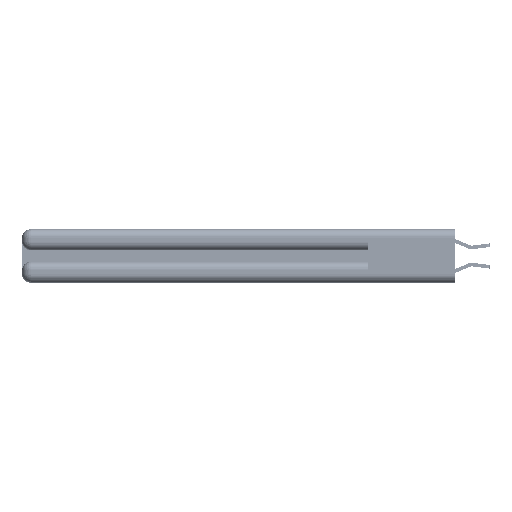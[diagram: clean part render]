
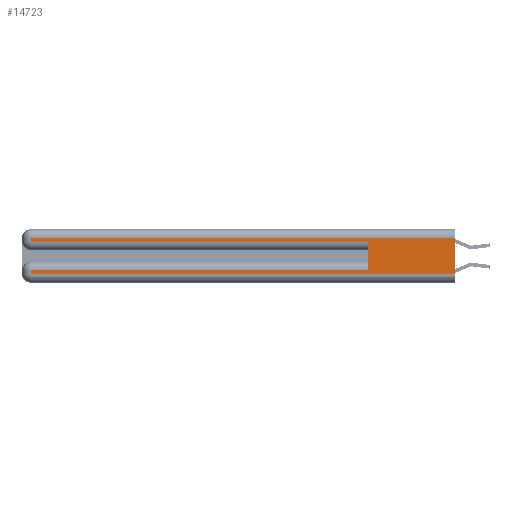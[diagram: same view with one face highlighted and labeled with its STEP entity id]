
A CAD part, left-side view. The second image highlights one B-rep face of the part: STEP entity #14723.
In plain terms, the highlighted planar face has unit normal (-1, 0, 0).
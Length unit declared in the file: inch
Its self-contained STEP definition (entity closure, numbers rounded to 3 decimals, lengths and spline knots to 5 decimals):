
#235 = LINE ( 'NONE', #29263, #10208 ) ;
#687 = ORIENTED_EDGE ( 'NONE', *, *, #10361, .T. ) ;
#1610 = CARTESIAN_POINT ( 'NONE',  ( 0., 2.94, 0.06 ) ) ;
#1762 = AXIS2_PLACEMENT_3D ( 'NONE', #10411, #19256, #21673 ) ;
#3569 = DIRECTION ( 'NONE',  ( 0., 0., 1. ) ) ;
#3870 = CARTESIAN_POINT ( 'NONE',  ( 0., 0., 0.06 ) ) ;
#4331 = CARTESIAN_POINT ( 'NONE',  ( 0., 0., 0.31 ) ) ;
#4814 = LINE ( 'NONE', #35301, #12497 ) ;
#5227 = PLANE ( 'NONE',  #1762 ) ;
#6048 = VERTEX_POINT ( 'NONE', #3870 ) ;
#6277 = VECTOR ( 'NONE', #28723, 39.37008 ) ;
#6961 = VECTOR ( 'NONE', #18670, 39.37008 ) ;
#7392 = CARTESIAN_POINT ( 'NONE',  ( 0., 0., 0.31 ) ) ;
#7670 = VERTEX_POINT ( 'NONE', #22877 ) ;
#8727 = EDGE_CURVE ( 'NONE', #21401, #6048, #20757, .T. ) ;
#8769 = VERTEX_POINT ( 'NONE', #32936 ) ;
#10208 = VECTOR ( 'NONE', #3569, 39.37008 ) ;
#10361 = EDGE_CURVE ( 'NONE', #26329, #7670, #27197, .T. ) ;
#10411 = CARTESIAN_POINT ( 'NONE',  ( 0., 0., 0.37 ) ) ;
#10543 = DIRECTION ( 'NONE',  ( 0., 1., 0. ) ) ;
#12447 = VECTOR ( 'NONE', #14994, 39.37008 ) ;
#12497 = VECTOR ( 'NONE', #15534, 39.37008 ) ;
#13702 = EDGE_CURVE ( 'NONE', #7670, #25701, #16628, .T. ) ;
#14043 = VERTEX_POINT ( 'NONE', #28996 ) ;
#14153 = ORIENTED_EDGE ( 'NONE', *, *, #13702, .T. ) ;
#14239 = LINE ( 'NONE', #19964, #19145 ) ;
#14723 = ADVANCED_FACE ( 'NONE', ( #33128 ), #5227, .F. ) ;
#14969 = EDGE_CURVE ( 'NONE', #8769, #21401, #18131, .T. ) ;
#14994 = DIRECTION ( 'NONE',  ( 0., 0., -1. ) ) ;
#15534 = DIRECTION ( 'NONE',  ( 0., 0., -1. ) ) ;
#15717 = CARTESIAN_POINT ( 'NONE',  ( 0., 2.94, 0.37 ) ) ;
#16628 = LINE ( 'NONE', #24954, #35956 ) ;
#17570 = EDGE_CURVE ( 'NONE', #14043, #35380, #235, .T. ) ;
#18131 = LINE ( 'NONE', #15717, #12447 ) ;
#18670 = DIRECTION ( 'NONE',  ( 0., 1., 0. ) ) ;
#19145 = VECTOR ( 'NONE', #31232, 39.37008 ) ;
#19256 = DIRECTION ( 'NONE',  ( 1., 0., 0. ) ) ;
#19964 = CARTESIAN_POINT ( 'NONE',  ( 0., 0., 0.285 ) ) ;
#20757 = LINE ( 'NONE', #32028, #6277 ) ;
#20929 = EDGE_CURVE ( 'NONE', #14043, #8769, #27363, .T. ) ;
#21401 = VERTEX_POINT ( 'NONE', #1610 ) ;
#21673 = DIRECTION ( 'NONE',  ( 0., 0., -1. ) ) ;
#21887 = ORIENTED_EDGE ( 'NONE', *, *, #35513, .T. ) ;
#22173 = DIRECTION ( 'NONE',  ( 0., 0., -1. ) ) ;
#22877 = CARTESIAN_POINT ( 'NONE',  ( 0., 2.94, 0.31 ) ) ;
#23595 = ORIENTED_EDGE ( 'NONE', *, *, #8727, .T. ) ;
#24398 = CARTESIAN_POINT ( 'NONE',  ( 0., 0., 0.085 ) ) ;
#24954 = CARTESIAN_POINT ( 'NONE',  ( 0., 2.94, 0.37 ) ) ;
#25662 = ORIENTED_EDGE ( 'NONE', *, *, #30347, .F. ) ;
#25701 = VERTEX_POINT ( 'NONE', #27200 ) ;
#26329 = VERTEX_POINT ( 'NONE', #4331 ) ;
#27197 = LINE ( 'NONE', #7392, #6961 ) ;
#27200 = CARTESIAN_POINT ( 'NONE',  ( 0., 2.94, 0.285 ) ) ;
#27363 = LINE ( 'NONE', #24398, #29256 ) ;
#27866 = ORIENTED_EDGE ( 'NONE', *, *, #20929, .T. ) ;
#28723 = DIRECTION ( 'NONE',  ( 0., -1., 0. ) ) ;
#28996 = CARTESIAN_POINT ( 'NONE',  ( 0., 0.6, 0.085 ) ) ;
#29256 = VECTOR ( 'NONE', #10543, 39.37008 ) ;
#29263 = CARTESIAN_POINT ( 'NONE',  ( 0., 0.6, 0.145 ) ) ;
#30347 = EDGE_CURVE ( 'NONE', #26329, #6048, #4814, .T. ) ;
#31232 = DIRECTION ( 'NONE',  ( 0., -1., 0. ) ) ;
#32028 = CARTESIAN_POINT ( 'NONE',  ( 0., 0., 0.06 ) ) ;
#32381 = EDGE_LOOP ( 'NONE', ( #25662, #687, #14153, #21887, #35373, #27866, #33283, #23595 ) ) ;
#32550 = CARTESIAN_POINT ( 'NONE',  ( 0., 0.6, 0.285 ) ) ;
#32936 = CARTESIAN_POINT ( 'NONE',  ( 0., 2.94, 0.085 ) ) ;
#33128 = FACE_OUTER_BOUND ( 'NONE', #32381, .T. ) ;
#33283 = ORIENTED_EDGE ( 'NONE', *, *, #14969, .T. ) ;
#35301 = CARTESIAN_POINT ( 'NONE',  ( 0., 0., 0.37 ) ) ;
#35373 = ORIENTED_EDGE ( 'NONE', *, *, #17570, .F. ) ;
#35380 = VERTEX_POINT ( 'NONE', #32550 ) ;
#35513 = EDGE_CURVE ( 'NONE', #25701, #35380, #14239, .T. ) ;
#35956 = VECTOR ( 'NONE', #22173, 39.37008 ) ;
